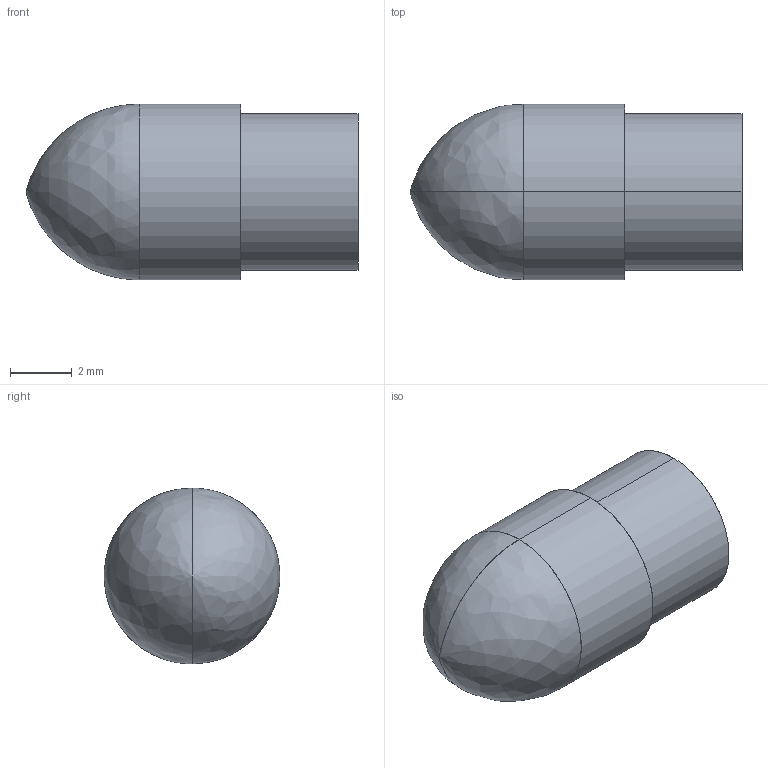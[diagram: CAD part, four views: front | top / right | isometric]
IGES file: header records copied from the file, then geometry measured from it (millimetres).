
Start section: SolidWorks IGES file using analytic representation for surfaces
Global section: file name: 22LR-Bullet.IGS; native system: SolidWorks 2011; preprocessor: SolidWorks 2011; author: Shane; date: 120428.213625; units: inch
Bounding box: 10.79 x 5.71 x 5.71 mm (x, y, z)
Surface area: 203.9 mm2 (no closed solid volume)
Topology: 0 solids, 0 shells, 8 faces, 120 edges, 118 vertices
Faces by surface type: bspline 4, revolution 4
